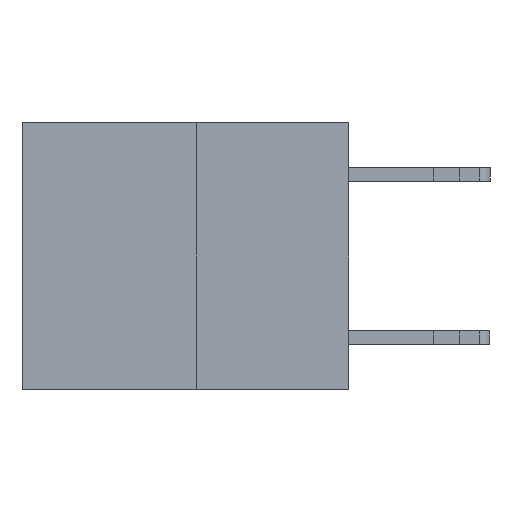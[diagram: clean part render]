
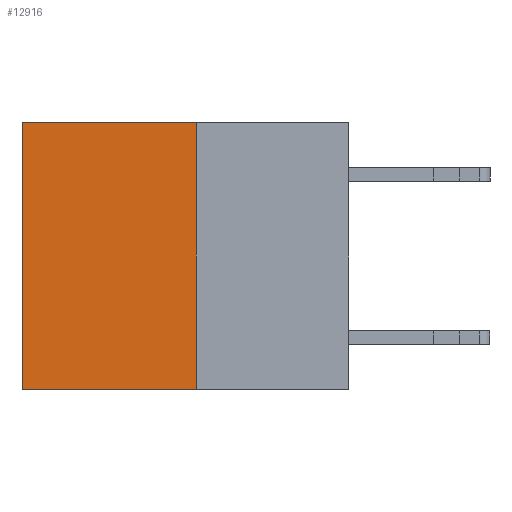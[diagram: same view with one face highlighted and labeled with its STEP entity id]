
A CAD part, left-side view. The second image highlights one B-rep face of the part: STEP entity #12916.
In plain terms, the highlighted planar face has unit normal (-1, 0, 0).
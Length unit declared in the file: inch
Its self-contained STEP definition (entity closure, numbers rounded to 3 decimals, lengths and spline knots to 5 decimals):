
#386 = DIRECTION ( 'NONE',  ( 1., 0., 0. ) ) ;
#1120 = VERTEX_POINT ( 'NONE', #7678 ) ;
#1380 = AXIS2_PLACEMENT_3D ( 'NONE', #3024, #386, #4410 ) ;
#1435 = EDGE_CURVE ( 'NONE', #10476, #1120, #8911, .T. ) ;
#1796 = DIRECTION ( 'NONE',  ( 0., 1., 0. ) ) ;
#2379 = VERTEX_POINT ( 'NONE', #14637 ) ;
#2552 = ORIENTED_EDGE ( 'NONE', *, *, #13722, .F. ) ;
#2670 = VECTOR ( 'NONE', #1796, 39.37008 ) ;
#3024 = CARTESIAN_POINT ( 'NONE',  ( 0.3165, 0.28, -0.49 ) ) ;
#4410 = DIRECTION ( 'NONE',  ( 0., 0., -1. ) ) ;
#5386 = VECTOR ( 'NONE', #12619, 39.37008 ) ;
#5548 = DIRECTION ( 'NONE',  ( 0., 0., -1. ) ) ;
#6278 = LINE ( 'NONE', #9820, #2670 ) ;
#6986 = DIRECTION ( 'NONE',  ( 0., 1., 0. ) ) ;
#7097 = CARTESIAN_POINT ( 'NONE',  ( 0.3165, 0.6, -0.49 ) ) ;
#7250 = EDGE_CURVE ( 'NONE', #2379, #11064, #15967, .T. ) ;
#7678 = CARTESIAN_POINT ( 'NONE',  ( 0.3165, 0.28, -0.49 ) ) ;
#8210 = CARTESIAN_POINT ( 'NONE',  ( 0.3165, 0.6, -0.49 ) ) ;
#8221 = ORIENTED_EDGE ( 'NONE', *, *, #1435, .F. ) ;
#8370 = PLANE ( 'NONE',  #1380 ) ;
#8645 = EDGE_CURVE ( 'NONE', #10476, #2379, #13465, .T. ) ;
#8911 = LINE ( 'NONE', #11382, #5386 ) ;
#9820 = CARTESIAN_POINT ( 'NONE',  ( 0.3165, 0.28, -0.49 ) ) ;
#9977 = EDGE_LOOP ( 'NONE', ( #15329, #2552, #8221, #13192 ) ) ;
#10031 = FACE_OUTER_BOUND ( 'NONE', #9977, .T. ) ;
#10476 = VERTEX_POINT ( 'NONE', #15973 ) ;
#10795 = VECTOR ( 'NONE', #6986, 39.37008 ) ;
#11064 = VERTEX_POINT ( 'NONE', #7097 ) ;
#11382 = CARTESIAN_POINT ( 'NONE',  ( 0.3165, 0.28, -0.49 ) ) ;
#12014 = VECTOR ( 'NONE', #5548, 39.37008 ) ;
#12619 = DIRECTION ( 'NONE',  ( 0., 0., -1. ) ) ;
#12916 = ADVANCED_FACE ( 'NONE', ( #10031 ), #8370, .F. ) ;
#13192 = ORIENTED_EDGE ( 'NONE', *, *, #8645, .T. ) ;
#13393 = CARTESIAN_POINT ( 'NONE',  ( 0.3165, 0.28, 0. ) ) ;
#13465 = LINE ( 'NONE', #13393, #10795 ) ;
#13722 = EDGE_CURVE ( 'NONE', #1120, #11064, #6278, .T. ) ;
#14637 = CARTESIAN_POINT ( 'NONE',  ( 0.3165, 0.6, 0. ) ) ;
#15329 = ORIENTED_EDGE ( 'NONE', *, *, #7250, .T. ) ;
#15967 = LINE ( 'NONE', #8210, #12014 ) ;
#15973 = CARTESIAN_POINT ( 'NONE',  ( 0.3165, 0.28, 0. ) ) ;
